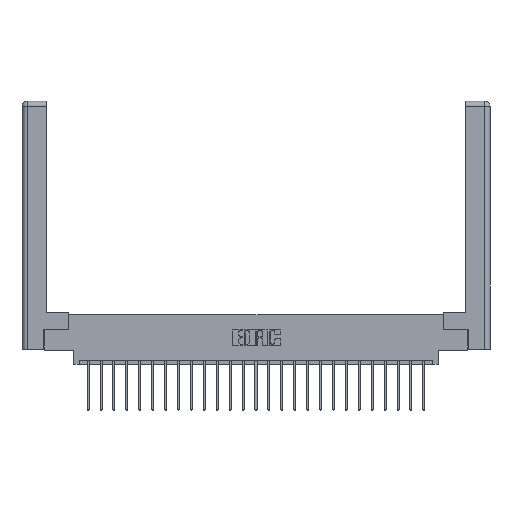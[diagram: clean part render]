
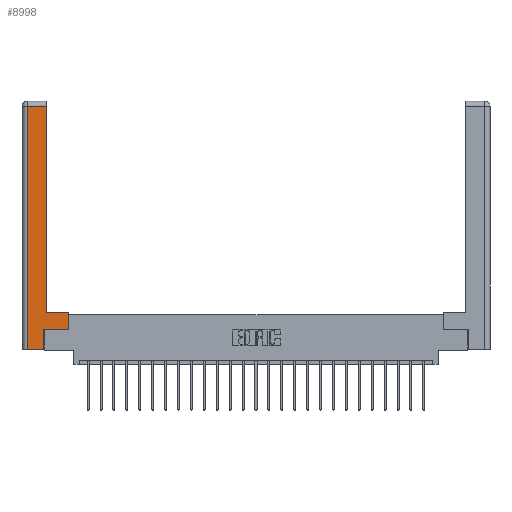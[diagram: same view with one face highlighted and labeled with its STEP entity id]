
A CAD part, top view. The second image highlights one B-rep face of the part: STEP entity #8998.
In plain terms, the highlighted planar face has unit normal (0, 0, 1).
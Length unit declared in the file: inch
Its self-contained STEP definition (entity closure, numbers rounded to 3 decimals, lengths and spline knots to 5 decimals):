
#94 = CARTESIAN_POINT ( 'NONE',  ( 0.295, 0.45, 0. ) ) ;
#106 = CARTESIAN_POINT ( 'NONE',  ( 0.265, 0., 0. ) ) ;
#123 = EDGE_CURVE ( 'NONE', #13351, #8025, #20235, .T. ) ;
#238 = VECTOR ( 'NONE', #14111, 39.37008 ) ;
#422 = CARTESIAN_POINT ( 'NONE',  ( 0.265, 0., 0. ) ) ;
#859 = EDGE_CURVE ( 'NONE', #23148, #8489, #21712, .T. ) ;
#934 = CARTESIAN_POINT ( 'NONE',  ( 0.295, 3., 0. ) ) ;
#1054 = CARTESIAN_POINT ( 'NONE',  ( 0.565, 0.245, 0. ) ) ;
#1135 = EDGE_CURVE ( 'NONE', #8489, #18144, #4727, .T. ) ;
#1139 = CARTESIAN_POINT ( 'NONE',  ( 0.265, 0.245, 0. ) ) ;
#1404 = FACE_OUTER_BOUND ( 'NONE', #13096, .T. ) ;
#1975 = VERTEX_POINT ( 'NONE', #422 ) ;
#2010 = VECTOR ( 'NONE', #20832, 39.37008 ) ;
#2083 = DIRECTION ( 'NONE',  ( 1., 0., 0. ) ) ;
#3038 = EDGE_CURVE ( 'NONE', #5086, #23148, #7052, .T. ) ;
#3450 = AXIS2_PLACEMENT_3D ( 'NONE', #20426, #22420, #24388 ) ;
#3570 = VECTOR ( 'NONE', #2083, 39.37008 ) ;
#3652 = DIRECTION ( 'NONE',  ( -1., 0., 0. ) ) ;
#4727 = LINE ( 'NONE', #934, #19937 ) ;
#4827 = VERTEX_POINT ( 'NONE', #6152 ) ;
#5086 = VERTEX_POINT ( 'NONE', #15500 ) ;
#5100 = LINE ( 'NONE', #106, #3570 ) ;
#6152 = CARTESIAN_POINT ( 'NONE',  ( 0.265, 0.245, 0. ) ) ;
#6352 = ORIENTED_EDGE ( 'NONE', *, *, #859, .T. ) ;
#6616 = ORIENTED_EDGE ( 'NONE', *, *, #19713, .T. ) ;
#6719 = ORIENTED_EDGE ( 'NONE', *, *, #1135, .T. ) ;
#7052 = LINE ( 'NONE', #10079, #238 ) ;
#7221 = ORIENTED_EDGE ( 'NONE', *, *, #24219, .T. ) ;
#7779 = VECTOR ( 'NONE', #13068, 39.37008 ) ;
#8025 = VERTEX_POINT ( 'NONE', #15620 ) ;
#8489 = VERTEX_POINT ( 'NONE', #94 ) ;
#8998 = ADVANCED_FACE ( 'NONE', ( #1404 ), #10567, .F. ) ;
#9151 = ORIENTED_EDGE ( 'NONE', *, *, #21344, .T. ) ;
#9474 = CARTESIAN_POINT ( 'NONE',  ( 0.0615, 2.94, 0. ) ) ;
#10079 = CARTESIAN_POINT ( 'NONE',  ( 0.565, 0.45, 0. ) ) ;
#10391 = VECTOR ( 'NONE', #3652, 39.37008 ) ;
#10567 = PLANE ( 'NONE',  #3450 ) ;
#11900 = DIRECTION ( 'NONE',  ( 0., -1., 0. ) ) ;
#12748 = VECTOR ( 'NONE', #19551, 39.37008 ) ;
#13068 = DIRECTION ( 'NONE',  ( 0., 1., 0. ) ) ;
#13096 = EDGE_LOOP ( 'NONE', ( #6719, #24503, #23383, #7221, #9151, #6616, #18521, #6352 ) ) ;
#13108 = CARTESIAN_POINT ( 'NONE',  ( 0.0615, 2.94, 0. ) ) ;
#13351 = VERTEX_POINT ( 'NONE', #13108 ) ;
#14111 = DIRECTION ( 'NONE',  ( 0., 1., 0. ) ) ;
#15500 = CARTESIAN_POINT ( 'NONE',  ( 0.565, 0.245, 0. ) ) ;
#15620 = CARTESIAN_POINT ( 'NONE',  ( 0.0615, 0., 0. ) ) ;
#15668 = LINE ( 'NONE', #9474, #10391 ) ;
#15901 = VECTOR ( 'NONE', #11900, 39.37008 ) ;
#18144 = VERTEX_POINT ( 'NONE', #23692 ) ;
#18521 = ORIENTED_EDGE ( 'NONE', *, *, #3038, .T. ) ;
#19551 = DIRECTION ( 'NONE',  ( -1., 0., 0. ) ) ;
#19713 = EDGE_CURVE ( 'NONE', #4827, #5086, #22501, .T. ) ;
#19937 = VECTOR ( 'NONE', #20544, 39.37008 ) ;
#20235 = LINE ( 'NONE', #23542, #15901 ) ;
#20426 = CARTESIAN_POINT ( 'NONE',  ( 0., 0., 0. ) ) ;
#20544 = DIRECTION ( 'NONE',  ( 0., 1., 0. ) ) ;
#20832 = DIRECTION ( 'NONE',  ( 1., 0., 0. ) ) ;
#21344 = EDGE_CURVE ( 'NONE', #1975, #4827, #25444, .T. ) ;
#21540 = CARTESIAN_POINT ( 'NONE',  ( 0.295, 0.45, 0. ) ) ;
#21712 = LINE ( 'NONE', #21540, #12748 ) ;
#22420 = DIRECTION ( 'NONE',  ( 0., 0., -1. ) ) ;
#22501 = LINE ( 'NONE', #1054, #2010 ) ;
#23148 = VERTEX_POINT ( 'NONE', #25485 ) ;
#23383 = ORIENTED_EDGE ( 'NONE', *, *, #123, .T. ) ;
#23542 = CARTESIAN_POINT ( 'NONE',  ( 0.0615, 0., 0. ) ) ;
#23692 = CARTESIAN_POINT ( 'NONE',  ( 0.295, 2.94, 0. ) ) ;
#24219 = EDGE_CURVE ( 'NONE', #8025, #1975, #5100, .T. ) ;
#24388 = DIRECTION ( 'NONE',  ( -1., 0., 0. ) ) ;
#24503 = ORIENTED_EDGE ( 'NONE', *, *, #24836, .T. ) ;
#24836 = EDGE_CURVE ( 'NONE', #18144, #13351, #15668, .T. ) ;
#25444 = LINE ( 'NONE', #1139, #7779 ) ;
#25485 = CARTESIAN_POINT ( 'NONE',  ( 0.565, 0.45, 0. ) ) ;
